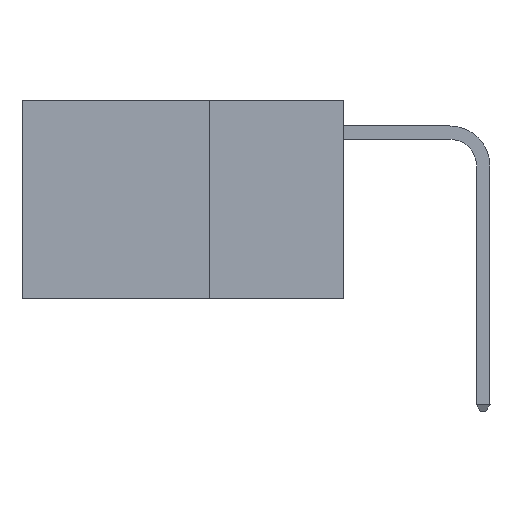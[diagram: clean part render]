
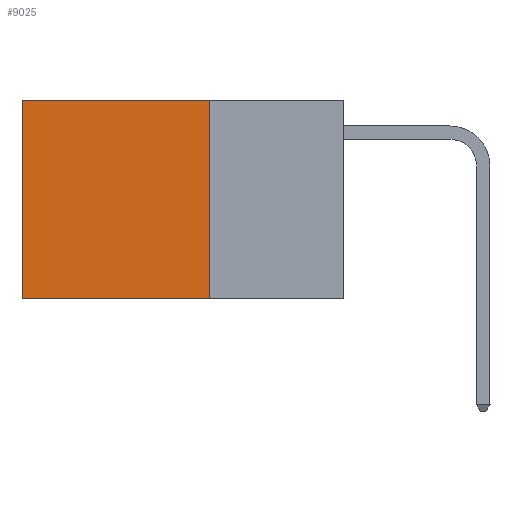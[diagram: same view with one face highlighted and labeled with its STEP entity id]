
A CAD part, left-side view. The second image highlights one B-rep face of the part: STEP entity #9025.
In plain terms, the highlighted planar face has unit normal (-1, 0, 0).
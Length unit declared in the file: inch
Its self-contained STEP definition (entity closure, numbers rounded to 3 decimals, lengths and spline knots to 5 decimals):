
#637 = CARTESIAN_POINT ( 'NONE',  ( 0.2625, 0.25, 0. ) ) ;
#723 = VECTOR ( 'NONE', #3206, 39.37008 ) ;
#787 = DIRECTION ( 'NONE',  ( 0., 1., 0. ) ) ;
#953 = AXIS2_PLACEMENT_3D ( 'NONE', #637, #1408, #6524 ) ;
#1286 = CARTESIAN_POINT ( 'NONE',  ( 0.2625, 0.25, 0. ) ) ;
#1331 = EDGE_CURVE ( 'NONE', #5762, #2169, #7914, .T. ) ;
#1408 = DIRECTION ( 'NONE',  ( 1., 0., 0. ) ) ;
#1418 = CARTESIAN_POINT ( 'NONE',  ( 0.2625, 0.25, 0. ) ) ;
#1847 = LINE ( 'NONE', #7322, #9229 ) ;
#2169 = VERTEX_POINT ( 'NONE', #5795 ) ;
#2705 = EDGE_CURVE ( 'NONE', #5762, #4627, #3770, .T. ) ;
#2910 = EDGE_CURVE ( 'NONE', #2169, #3580, #3882, .T. ) ;
#3206 = DIRECTION ( 'NONE',  ( 0., 1., 0. ) ) ;
#3580 = VERTEX_POINT ( 'NONE', #5339 ) ;
#3770 = LINE ( 'NONE', #1286, #5477 ) ;
#3882 = LINE ( 'NONE', #8158, #9289 ) ;
#4627 = VERTEX_POINT ( 'NONE', #7236 ) ;
#5088 = FACE_OUTER_BOUND ( 'NONE', #6753, .T. ) ;
#5339 = CARTESIAN_POINT ( 'NONE',  ( 0.2625, 0.6, -0.37 ) ) ;
#5477 = VECTOR ( 'NONE', #5691, 39.37008 ) ;
#5691 = DIRECTION ( 'NONE',  ( 0., 0., -1. ) ) ;
#5762 = VERTEX_POINT ( 'NONE', #6216 ) ;
#5795 = CARTESIAN_POINT ( 'NONE',  ( 0.2625, 0.6, 0. ) ) ;
#6216 = CARTESIAN_POINT ( 'NONE',  ( 0.2625, 0.25, 0. ) ) ;
#6524 = DIRECTION ( 'NONE',  ( 0., 0., -1. ) ) ;
#6743 = EDGE_CURVE ( 'NONE', #4627, #3580, #1847, .T. ) ;
#6746 = DIRECTION ( 'NONE',  ( 0., 0., -1. ) ) ;
#6753 = EDGE_LOOP ( 'NONE', ( #8198, #8093, #8946, #8651 ) ) ;
#7236 = CARTESIAN_POINT ( 'NONE',  ( 0.2625, 0.25, -0.37 ) ) ;
#7322 = CARTESIAN_POINT ( 'NONE',  ( 0.2625, 0.25, -0.37 ) ) ;
#7914 = LINE ( 'NONE', #1418, #723 ) ;
#8093 = ORIENTED_EDGE ( 'NONE', *, *, #6743, .F. ) ;
#8158 = CARTESIAN_POINT ( 'NONE',  ( 0.2625, 0.6, 0. ) ) ;
#8198 = ORIENTED_EDGE ( 'NONE', *, *, #2910, .T. ) ;
#8651 = ORIENTED_EDGE ( 'NONE', *, *, #1331, .T. ) ;
#8946 = ORIENTED_EDGE ( 'NONE', *, *, #2705, .F. ) ;
#9025 = ADVANCED_FACE ( 'NONE', ( #5088 ), #9258, .F. ) ;
#9229 = VECTOR ( 'NONE', #787, 39.37008 ) ;
#9258 = PLANE ( 'NONE',  #953 ) ;
#9289 = VECTOR ( 'NONE', #6746, 39.37008 ) ;
